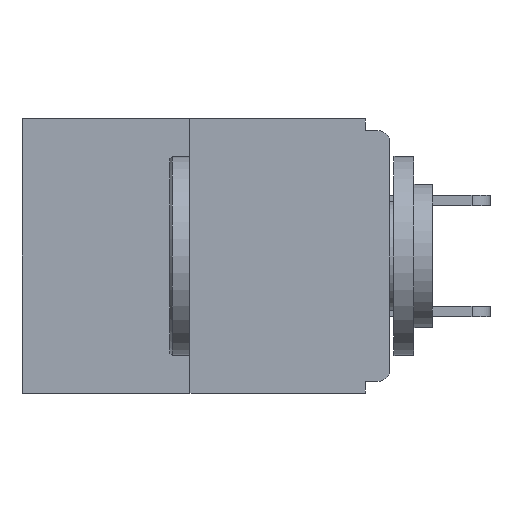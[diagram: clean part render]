
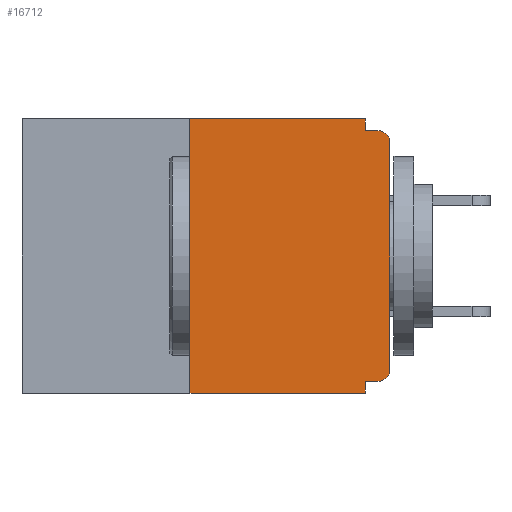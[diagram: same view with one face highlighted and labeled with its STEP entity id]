
A CAD part, left-side view. The second image highlights one B-rep face of the part: STEP entity #16712.
In plain terms, the highlighted planar face has unit normal (-1, 0, 0).
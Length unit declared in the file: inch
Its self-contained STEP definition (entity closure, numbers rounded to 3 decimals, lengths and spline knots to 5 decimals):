
#281 = DIRECTION ( 'NONE',  ( 1., 0., 0. ) ) ;
#368 = VERTEX_POINT ( 'NONE', #17312 ) ;
#1141 = LINE ( 'NONE', #8795, #9486 ) ;
#1240 = EDGE_CURVE ( 'NONE', #6343, #3442, #21779, .T. ) ;
#1369 = AXIS2_PLACEMENT_3D ( 'NONE', #2328, #281, #23320 ) ;
#1477 = AXIS2_PLACEMENT_3D ( 'NONE', #1531, #12967, #8521 ) ;
#1518 = DIRECTION ( 'NONE',  ( 0., 0., 1. ) ) ;
#1531 = CARTESIAN_POINT ( 'NONE',  ( 0., 0.015, -0.313 ) ) ;
#2021 = ORIENTED_EDGE ( 'NONE', *, *, #27142, .F. ) ;
#2103 = VECTOR ( 'NONE', #1518, 39.37008 ) ;
#2185 = EDGE_CURVE ( 'NONE', #22671, #13103, #24685, .T. ) ;
#2251 = VECTOR ( 'NONE', #28253, 39.37008 ) ;
#2328 = CARTESIAN_POINT ( 'NONE',  ( 0., 0.46, 0. ) ) ;
#3442 = VERTEX_POINT ( 'NONE', #27271 ) ;
#3675 = CARTESIAN_POINT ( 'NONE',  ( 0., 0.031, -0.328 ) ) ;
#3777 = CARTESIAN_POINT ( 'NONE',  ( 0., 0., -0.03 ) ) ;
#4706 = CARTESIAN_POINT ( 'NONE',  ( 0., 0.031, 0. ) ) ;
#4854 = ORIENTED_EDGE ( 'NONE', *, *, #2185, .F. ) ;
#5825 = DIRECTION ( 'NONE',  ( 0., 0., -1. ) ) ;
#6169 = DIRECTION ( 'NONE',  ( 0., -1., 0. ) ) ;
#6343 = VERTEX_POINT ( 'NONE', #3777 ) ;
#7372 = ORIENTED_EDGE ( 'NONE', *, *, #26099, .T. ) ;
#7627 = CARTESIAN_POINT ( 'NONE',  ( 0., 0.25, 0. ) ) ;
#8211 = CARTESIAN_POINT ( 'NONE',  ( 0., 0.46, 0. ) ) ;
#8508 = CARTESIAN_POINT ( 'NONE',  ( 0., 0.015, -0.328 ) ) ;
#8521 = DIRECTION ( 'NONE',  ( 0., 0., -1. ) ) ;
#8702 = DIRECTION ( 'NONE',  ( 0., -1., 0. ) ) ;
#8795 = CARTESIAN_POINT ( 'NONE',  ( 0., 0., -0.015 ) ) ;
#9486 = VECTOR ( 'NONE', #8702, 39.37008 ) ;
#10165 = VECTOR ( 'NONE', #20276, 39.37008 ) ;
#10691 = VECTOR ( 'NONE', #11208, 39.37008 ) ;
#10926 = EDGE_CURVE ( 'NONE', #22376, #26367, #16320, .T. ) ;
#11208 = DIRECTION ( 'NONE',  ( 0., 0., -1. ) ) ;
#11656 = CARTESIAN_POINT ( 'NONE',  ( 0., 0.015, -0.03 ) ) ;
#12029 = CARTESIAN_POINT ( 'NONE',  ( 0., 0., 0. ) ) ;
#12967 = DIRECTION ( 'NONE',  ( -1., 0., 0. ) ) ;
#13103 = VERTEX_POINT ( 'NONE', #4706 ) ;
#14075 = CARTESIAN_POINT ( 'NONE',  ( 0., 0., -0.313 ) ) ;
#14169 = VERTEX_POINT ( 'NONE', #24756 ) ;
#14455 = AXIS2_PLACEMENT_3D ( 'NONE', #11656, #25512, #23262 ) ;
#15289 = EDGE_CURVE ( 'NONE', #368, #22671, #27546, .T. ) ;
#15379 = ORIENTED_EDGE ( 'NONE', *, *, #10926, .F. ) ;
#16184 = PLANE ( 'NONE',  #1369 ) ;
#16320 = LINE ( 'NONE', #19971, #10165 ) ;
#16340 = LINE ( 'NONE', #25732, #2251 ) ;
#16712 = ADVANCED_FACE ( 'NONE', ( #25270 ), #16184, .F. ) ;
#16850 = LINE ( 'NONE', #25054, #10691 ) ;
#17312 = CARTESIAN_POINT ( 'NONE',  ( 0., 0.25, -0.343 ) ) ;
#17565 = VECTOR ( 'NONE', #28526, 39.37008 ) ;
#18626 = ORIENTED_EDGE ( 'NONE', *, *, #15289, .F. ) ;
#19042 = CIRCLE ( 'NONE', #1477, 0.015 ) ;
#19304 = VERTEX_POINT ( 'NONE', #23896 ) ;
#19971 = CARTESIAN_POINT ( 'NONE',  ( 0., 0., -0.328 ) ) ;
#20276 = DIRECTION ( 'NONE',  ( 0., 1., 0. ) ) ;
#20512 = ORIENTED_EDGE ( 'NONE', *, *, #24888, .T. ) ;
#20951 = EDGE_LOOP ( 'NONE', ( #4854, #18626, #7372, #2021, #15379, #20512, #29944, #26469, #28848, #25790 ) ) ;
#21779 = CIRCLE ( 'NONE', #14455, 0.015 ) ;
#22294 = LINE ( 'NONE', #12029, #17565 ) ;
#22376 = VERTEX_POINT ( 'NONE', #8508 ) ;
#22671 = VERTEX_POINT ( 'NONE', #7627 ) ;
#23262 = DIRECTION ( 'NONE',  ( 0., 0., -1. ) ) ;
#23320 = DIRECTION ( 'NONE',  ( 0., 0., -1. ) ) ;
#23576 = VECTOR ( 'NONE', #6169, 39.37008 ) ;
#23896 = CARTESIAN_POINT ( 'NONE',  ( 0., 0.031, -0.343 ) ) ;
#24347 = CARTESIAN_POINT ( 'NONE',  ( 0., 0.031, 0. ) ) ;
#24685 = LINE ( 'NONE', #8211, #23576 ) ;
#24756 = CARTESIAN_POINT ( 'NONE',  ( 0., 0.031, -0.015 ) ) ;
#24888 = EDGE_CURVE ( 'NONE', #22376, #29968, #19042, .T. ) ;
#25054 = CARTESIAN_POINT ( 'NONE',  ( 0., 0.031, -0.343 ) ) ;
#25185 = EDGE_CURVE ( 'NONE', #29968, #6343, #22294, .T. ) ;
#25270 = FACE_OUTER_BOUND ( 'NONE', #20951, .T. ) ;
#25347 = EDGE_CURVE ( 'NONE', #13103, #14169, #28813, .T. ) ;
#25512 = DIRECTION ( 'NONE',  ( -1., 0., 0. ) ) ;
#25732 = CARTESIAN_POINT ( 'NONE',  ( 0., 0.46, -0.343 ) ) ;
#25790 = ORIENTED_EDGE ( 'NONE', *, *, #25347, .F. ) ;
#26099 = EDGE_CURVE ( 'NONE', #368, #19304, #16340, .T. ) ;
#26367 = VERTEX_POINT ( 'NONE', #3675 ) ;
#26469 = ORIENTED_EDGE ( 'NONE', *, *, #1240, .T. ) ;
#27131 = CARTESIAN_POINT ( 'NONE',  ( 0., 0.25, 0. ) ) ;
#27142 = EDGE_CURVE ( 'NONE', #26367, #19304, #16850, .T. ) ;
#27271 = CARTESIAN_POINT ( 'NONE',  ( 0., 0.015, -0.015 ) ) ;
#27546 = LINE ( 'NONE', #27131, #2103 ) ;
#28253 = DIRECTION ( 'NONE',  ( 0., -1., 0. ) ) ;
#28456 = VECTOR ( 'NONE', #5825, 39.37008 ) ;
#28526 = DIRECTION ( 'NONE',  ( 0., 0., 1. ) ) ;
#28593 = EDGE_CURVE ( 'NONE', #14169, #3442, #1141, .T. ) ;
#28813 = LINE ( 'NONE', #24347, #28456 ) ;
#28848 = ORIENTED_EDGE ( 'NONE', *, *, #28593, .F. ) ;
#29944 = ORIENTED_EDGE ( 'NONE', *, *, #25185, .T. ) ;
#29968 = VERTEX_POINT ( 'NONE', #14075 ) ;
